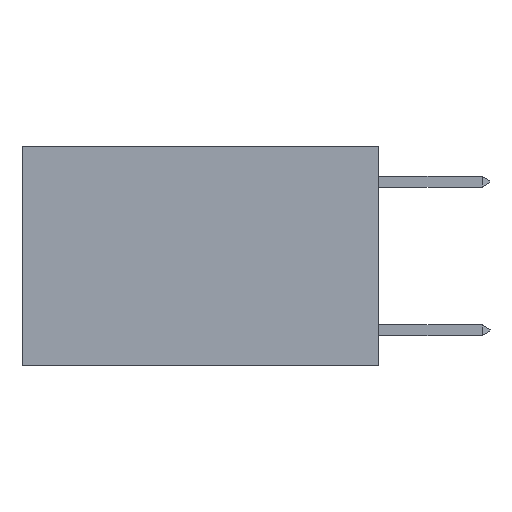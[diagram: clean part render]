
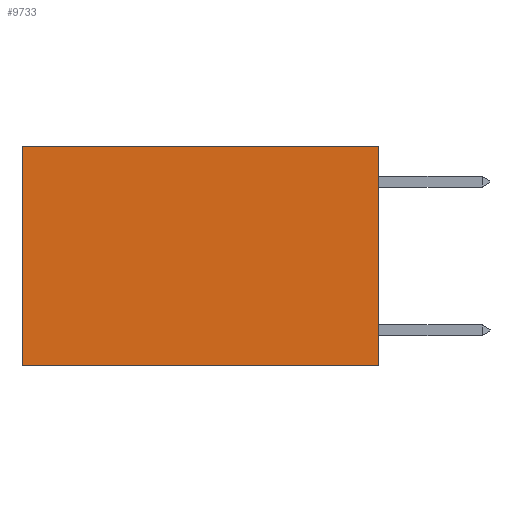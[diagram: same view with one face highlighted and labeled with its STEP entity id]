
A CAD part, left-side view. The second image highlights one B-rep face of the part: STEP entity #9733.
In plain terms, the highlighted planar face has unit normal (-1, 0, 0).
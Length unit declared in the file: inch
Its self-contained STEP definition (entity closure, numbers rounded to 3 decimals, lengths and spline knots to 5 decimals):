
#1281 = DIRECTION ( 'NONE',  ( 1., 0., 0. ) ) ;
#1537 = EDGE_CURVE ( 'NONE', #17013, #15562, #16457, .T. ) ;
#3791 = CARTESIAN_POINT ( 'NONE',  ( 0.2625, 0.6, 0. ) ) ;
#3882 = ORIENTED_EDGE ( 'NONE', *, *, #1537, .T. ) ;
#4837 = ORIENTED_EDGE ( 'NONE', *, *, #17877, .F. ) ;
#4925 = VERTEX_POINT ( 'NONE', #15540 ) ;
#5426 = VECTOR ( 'NONE', #13577, 39.37008 ) ;
#5440 = LINE ( 'NONE', #6505, #19611 ) ;
#6505 = CARTESIAN_POINT ( 'NONE',  ( 0.2625, 0., 0. ) ) ;
#8088 = VERTEX_POINT ( 'NONE', #9357 ) ;
#9357 = CARTESIAN_POINT ( 'NONE',  ( 0.2625, 0.6, -0.37 ) ) ;
#9699 = DIRECTION ( 'NONE',  ( 0., 0., -1. ) ) ;
#9733 = ADVANCED_FACE ( 'NONE', ( #11807 ), #17085, .F. ) ;
#9788 = EDGE_CURVE ( 'NONE', #15562, #8088, #18477, .T. ) ;
#10157 = LINE ( 'NONE', #13639, #5426 ) ;
#10792 = CARTESIAN_POINT ( 'NONE',  ( 0.2625, 0., 0. ) ) ;
#11190 = CARTESIAN_POINT ( 'NONE',  ( 0.2625, 0.6, 0. ) ) ;
#11807 = FACE_OUTER_BOUND ( 'NONE', #13353, .T. ) ;
#13353 = EDGE_LOOP ( 'NONE', ( #15658, #4837, #16988, #3882 ) ) ;
#13577 = DIRECTION ( 'NONE',  ( 0., 1., 0. ) ) ;
#13639 = CARTESIAN_POINT ( 'NONE',  ( 0.2625, 0., -0.37 ) ) ;
#14387 = DIRECTION ( 'NONE',  ( 0., 0., -1. ) ) ;
#15540 = CARTESIAN_POINT ( 'NONE',  ( 0.2625, 0., -0.37 ) ) ;
#15562 = VERTEX_POINT ( 'NONE', #3791 ) ;
#15655 = CARTESIAN_POINT ( 'NONE',  ( 0.2625, 0., 0. ) ) ;
#15658 = ORIENTED_EDGE ( 'NONE', *, *, #9788, .T. ) ;
#16457 = LINE ( 'NONE', #15655, #18950 ) ;
#16988 = ORIENTED_EDGE ( 'NONE', *, *, #17720, .F. ) ;
#17013 = VERTEX_POINT ( 'NONE', #19042 ) ;
#17085 = PLANE ( 'NONE',  #18699 ) ;
#17125 = DIRECTION ( 'NONE',  ( 0., 1., 0. ) ) ;
#17477 = VECTOR ( 'NONE', #14387, 39.37008 ) ;
#17720 = EDGE_CURVE ( 'NONE', #17013, #4925, #5440, .T. ) ;
#17877 = EDGE_CURVE ( 'NONE', #4925, #8088, #10157, .T. ) ;
#18477 = LINE ( 'NONE', #11190, #17477 ) ;
#18699 = AXIS2_PLACEMENT_3D ( 'NONE', #10792, #1281, #18768 ) ;
#18768 = DIRECTION ( 'NONE',  ( 0., 0., -1. ) ) ;
#18950 = VECTOR ( 'NONE', #17125, 39.37008 ) ;
#19042 = CARTESIAN_POINT ( 'NONE',  ( 0.2625, 0., 0. ) ) ;
#19611 = VECTOR ( 'NONE', #9699, 39.37008 ) ;
